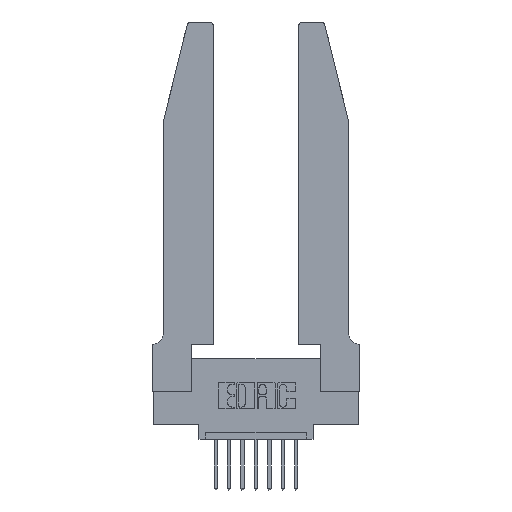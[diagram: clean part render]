
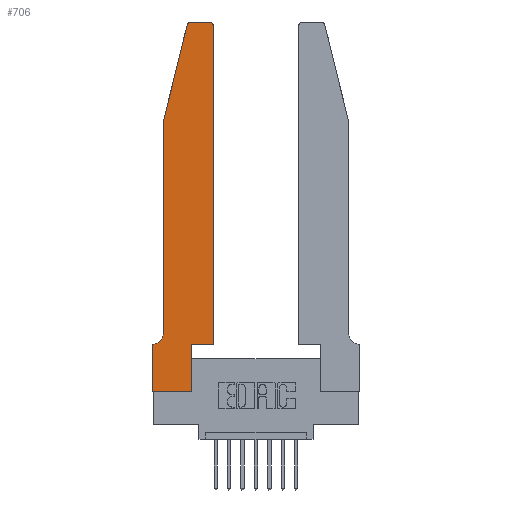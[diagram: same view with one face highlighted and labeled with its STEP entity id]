
A CAD part, top view. The second image highlights one B-rep face of the part: STEP entity #706.
In plain terms, the highlighted planar face has unit normal (0, 0, 1).
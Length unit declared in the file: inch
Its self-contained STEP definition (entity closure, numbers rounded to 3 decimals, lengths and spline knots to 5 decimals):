
#121 = CARTESIAN_POINT ( 'NONE',  ( 0., 0.35, 0.37 ) ) ;
#126 = VERTEX_POINT ( 'NONE', #1952 ) ;
#167 = FACE_OUTER_BOUND ( 'NONE', #6563, .T. ) ;
#379 = DIRECTION ( 'NONE',  ( 0., -1., 0. ) ) ;
#645 = ORIENTED_EDGE ( 'NONE', *, *, #4341, .T. ) ;
#706 = ADVANCED_FACE ( 'NONE', ( #167 ), #10899, .T. ) ;
#739 = CARTESIAN_POINT ( 'NONE',  ( 0.2865, 0.35, 0.37 ) ) ;
#1592 = ORIENTED_EDGE ( 'NONE', *, *, #12688, .T. ) ;
#1952 = CARTESIAN_POINT ( 'NONE',  ( 0.0755, 0.42, 0.37 ) ) ;
#1966 = ORIENTED_EDGE ( 'NONE', *, *, #12650, .T. ) ;
#2096 = VERTEX_POINT ( 'NONE', #11138 ) ;
#2237 = EDGE_CURVE ( 'NONE', #8743, #3703, #14157, .T. ) ;
#2288 = CIRCLE ( 'NONE', #3729, 0.03 ) ;
#2378 = DIRECTION ( 'NONE',  ( -1., 0., 0. ) ) ;
#2755 = VERTEX_POINT ( 'NONE', #7861 ) ;
#2904 = VERTEX_POINT ( 'NONE', #6020 ) ;
#2953 = ORIENTED_EDGE ( 'NONE', *, *, #8154, .T. ) ;
#3117 = CARTESIAN_POINT ( 'NONE',  ( 0.2865, 0., 0.37 ) ) ;
#3230 = EDGE_CURVE ( 'NONE', #2904, #4350, #9642, .T. ) ;
#3308 = DIRECTION ( 'NONE',  ( 0., 0., 1. ) ) ;
#3536 = AXIS2_PLACEMENT_3D ( 'NONE', #12167, #13359, #6481 ) ;
#3615 = VERTEX_POINT ( 'NONE', #7773 ) ;
#3703 = VERTEX_POINT ( 'NONE', #3117 ) ;
#3729 = AXIS2_PLACEMENT_3D ( 'NONE', #6294, #10797, #9658 ) ;
#3889 = VECTOR ( 'NONE', #2378, 39.37008 ) ;
#3912 = CARTESIAN_POINT ( 'NONE',  ( 0.0755, 2., 0.37 ) ) ;
#4341 = EDGE_CURVE ( 'NONE', #5580, #5387, #10708, .T. ) ;
#4350 = VERTEX_POINT ( 'NONE', #5086 ) ;
#4456 = VECTOR ( 'NONE', #6492, 39.37008 ) ;
#4468 = ORIENTED_EDGE ( 'NONE', *, *, #10826, .T. ) ;
#4609 = CIRCLE ( 'NONE', #11645, 0.03 ) ;
#4857 = CARTESIAN_POINT ( 'NONE',  ( 0.25487, 2.72718, 0.37 ) ) ;
#5086 = CARTESIAN_POINT ( 'NONE',  ( 0.284, 2.75, 0.37 ) ) ;
#5132 = CARTESIAN_POINT ( 'NONE',  ( 0., 0.35, 0.37 ) ) ;
#5365 = VERTEX_POINT ( 'NONE', #11404 ) ;
#5382 = CARTESIAN_POINT ( 'NONE',  ( 0.0755, 2., 0.37 ) ) ;
#5387 = VERTEX_POINT ( 'NONE', #121 ) ;
#5580 = VERTEX_POINT ( 'NONE', #8863 ) ;
#5925 = LINE ( 'NONE', #3912, #12364 ) ;
#5937 = VECTOR ( 'NONE', #10444, 39.37008 ) ;
#6020 = CARTESIAN_POINT ( 'NONE',  ( 0.4205, 2.75, 0.37 ) ) ;
#6294 = CARTESIAN_POINT ( 'NONE',  ( 0.4205, 2.72, 0.37 ) ) ;
#6351 = CARTESIAN_POINT ( 'NONE',  ( 0., 0., 0.37 ) ) ;
#6355 = ORIENTED_EDGE ( 'NONE', *, *, #12323, .T. ) ;
#6481 = DIRECTION ( 'NONE',  ( -1., 0., 0. ) ) ;
#6492 = DIRECTION ( 'NONE',  ( -0.239, -0.971, 0. ) ) ;
#6563 = EDGE_LOOP ( 'NONE', ( #14361, #14384, #6355, #1592, #13022, #645, #2953, #13516, #12259, #4468, #13545, #1966 ) ) ;
#6650 = LINE ( 'NONE', #739, #9018 ) ;
#7012 = LINE ( 'NONE', #9340, #5937 ) ;
#7417 = CARTESIAN_POINT ( 'NONE',  ( 0.0755, 0.35, 0.37 ) ) ;
#7512 = DIRECTION ( 'NONE',  ( 1., 0., 0. ) ) ;
#7563 = DIRECTION ( 'NONE',  ( 0., 0., 1. ) ) ;
#7773 = CARTESIAN_POINT ( 'NONE',  ( 0.4505, 0.35, 0.37 ) ) ;
#7861 = CARTESIAN_POINT ( 'NONE',  ( 0.2865, 0.35, 0.37 ) ) ;
#7954 = EDGE_CURVE ( 'NONE', #3703, #2755, #6650, .T. ) ;
#8078 = CARTESIAN_POINT ( 'NONE',  ( 0.284, 2.72, 0.37 ) ) ;
#8080 = VECTOR ( 'NONE', #14383, 39.37008 ) ;
#8154 = EDGE_CURVE ( 'NONE', #5387, #8743, #10247, .T. ) ;
#8515 = DIRECTION ( 'NONE',  ( 0., 1., 0. ) ) ;
#8743 = VERTEX_POINT ( 'NONE', #14815 ) ;
#8863 = CARTESIAN_POINT ( 'NONE',  ( 0.0055, 0.35, 0.37 ) ) ;
#9018 = VECTOR ( 'NONE', #8515, 39.37008 ) ;
#9279 = CARTESIAN_POINT ( 'NONE',  ( 0.2605, 2.75, 0.37 ) ) ;
#9340 = CARTESIAN_POINT ( 'NONE',  ( 0.4505, 0.35, 0.37 ) ) ;
#9642 = LINE ( 'NONE', #9279, #3889 ) ;
#9658 = DIRECTION ( 'NONE',  ( 1., 0., 0. ) ) ;
#9760 = DIRECTION ( 'NONE',  ( -1., 0., 0. ) ) ;
#10159 = CARTESIAN_POINT ( 'NONE',  ( 0.4505, 0.35, 0.37 ) ) ;
#10247 = LINE ( 'NONE', #11897, #12048 ) ;
#10444 = DIRECTION ( 'NONE',  ( 0., 1., 0. ) ) ;
#10612 = LINE ( 'NONE', #10159, #11332 ) ;
#10708 = LINE ( 'NONE', #7417, #11236 ) ;
#10797 = DIRECTION ( 'NONE',  ( 0., 0., 1. ) ) ;
#10826 = EDGE_CURVE ( 'NONE', #2755, #3615, #10612, .T. ) ;
#10899 = PLANE ( 'NONE',  #14394 ) ;
#11138 = CARTESIAN_POINT ( 'NONE',  ( 0.0755, 2., 0.37 ) ) ;
#11161 = EDGE_CURVE ( 'NONE', #126, #5580, #14733, .T. ) ;
#11236 = VECTOR ( 'NONE', #9760, 39.37008 ) ;
#11291 = LINE ( 'NONE', #5382, #4456 ) ;
#11332 = VECTOR ( 'NONE', #12539, 39.37008 ) ;
#11356 = DIRECTION ( 'NONE',  ( 1., 0., 0. ) ) ;
#11404 = CARTESIAN_POINT ( 'NONE',  ( 0.4505, 2.72, 0.37 ) ) ;
#11645 = AXIS2_PLACEMENT_3D ( 'NONE', #8078, #3308, #11356 ) ;
#11897 = CARTESIAN_POINT ( 'NONE',  ( 0., 0., 0.37 ) ) ;
#11916 = EDGE_CURVE ( 'NONE', #3615, #5365, #7012, .T. ) ;
#12024 = DIRECTION ( 'NONE',  ( 0., -1., 0. ) ) ;
#12048 = VECTOR ( 'NONE', #379, 39.37008 ) ;
#12167 = CARTESIAN_POINT ( 'NONE',  ( 0.0055, 0.42, 0.37 ) ) ;
#12259 = ORIENTED_EDGE ( 'NONE', *, *, #7954, .T. ) ;
#12323 = EDGE_CURVE ( 'NONE', #13108, #2096, #11291, .T. ) ;
#12364 = VECTOR ( 'NONE', #12024, 39.37008 ) ;
#12539 = DIRECTION ( 'NONE',  ( 1., 0., 0. ) ) ;
#12650 = EDGE_CURVE ( 'NONE', #5365, #2904, #2288, .T. ) ;
#12688 = EDGE_CURVE ( 'NONE', #2096, #126, #5925, .T. ) ;
#13022 = ORIENTED_EDGE ( 'NONE', *, *, #11161, .T. ) ;
#13108 = VERTEX_POINT ( 'NONE', #4857 ) ;
#13359 = DIRECTION ( 'NONE',  ( 0., 0., -1. ) ) ;
#13368 = EDGE_CURVE ( 'NONE', #4350, #13108, #4609, .T. ) ;
#13516 = ORIENTED_EDGE ( 'NONE', *, *, #2237, .T. ) ;
#13545 = ORIENTED_EDGE ( 'NONE', *, *, #11916, .T. ) ;
#14157 = LINE ( 'NONE', #6351, #8080 ) ;
#14361 = ORIENTED_EDGE ( 'NONE', *, *, #3230, .T. ) ;
#14384 = ORIENTED_EDGE ( 'NONE', *, *, #13368, .T. ) ;
#14383 = DIRECTION ( 'NONE',  ( 1., 0., 0. ) ) ;
#14394 = AXIS2_PLACEMENT_3D ( 'NONE', #5132, #7563, #7512 ) ;
#14733 = CIRCLE ( 'NONE', #3536, 0.07 ) ;
#14815 = CARTESIAN_POINT ( 'NONE',  ( 0., 0., 0.37 ) ) ;
